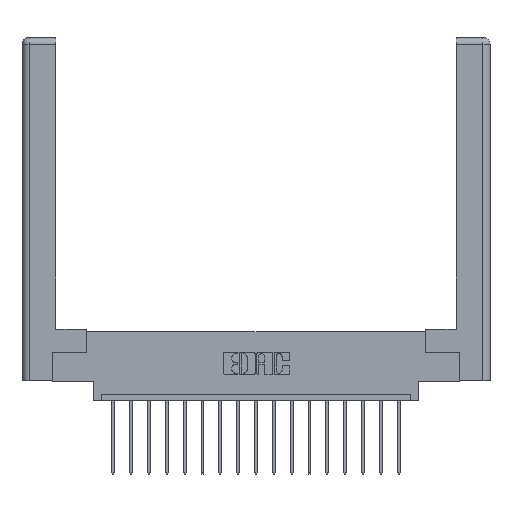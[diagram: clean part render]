
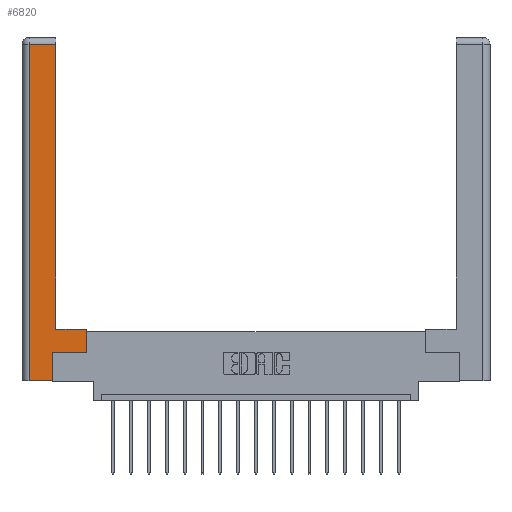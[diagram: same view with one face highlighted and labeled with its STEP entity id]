
A CAD part, top view. The second image highlights one B-rep face of the part: STEP entity #6820.
In plain terms, the highlighted planar face has unit normal (0, 0, 1).
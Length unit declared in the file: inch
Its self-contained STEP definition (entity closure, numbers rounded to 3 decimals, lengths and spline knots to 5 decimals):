
#52 = EDGE_CURVE ( 'NONE', #8139, #12732, #12989, .T. ) ;
#193 = DIRECTION ( 'NONE',  ( -1., 0., 0. ) ) ;
#220 = CARTESIAN_POINT ( 'NONE',  ( 0.565, 0.45, 0. ) ) ;
#452 = DIRECTION ( 'NONE',  ( 0., 1., 0. ) ) ;
#694 = EDGE_CURVE ( 'NONE', #10817, #9784, #9829, .T. ) ;
#1513 = VECTOR ( 'NONE', #9734, 39.37008 ) ;
#1611 = CARTESIAN_POINT ( 'NONE',  ( 0.295, 0.45, 0. ) ) ;
#1675 = ORIENTED_EDGE ( 'NONE', *, *, #2517, .T. ) ;
#1858 = VERTEX_POINT ( 'NONE', #13927 ) ;
#2036 = ORIENTED_EDGE ( 'NONE', *, *, #6158, .T. ) ;
#2280 = VECTOR ( 'NONE', #14547, 39.37008 ) ;
#2361 = EDGE_CURVE ( 'NONE', #12071, #10817, #10763, .T. ) ;
#2517 = EDGE_CURVE ( 'NONE', #3323, #8139, #18394, .T. ) ;
#2618 = VECTOR ( 'NONE', #4330, 39.37008 ) ;
#2687 = CARTESIAN_POINT ( 'NONE',  ( 0.265, 0., 0. ) ) ;
#3151 = EDGE_LOOP ( 'NONE', ( #13550, #15215, #8294, #9806, #11134, #3473, #2036, #1675 ) ) ;
#3323 = VERTEX_POINT ( 'NONE', #18029 ) ;
#3473 = ORIENTED_EDGE ( 'NONE', *, *, #9167, .T. ) ;
#3903 = DIRECTION ( 'NONE',  ( -1., 0., 0. ) ) ;
#3981 = DIRECTION ( 'NONE',  ( 0., -1., 0. ) ) ;
#4330 = DIRECTION ( 'NONE',  ( -1., 0., 0. ) ) ;
#4354 = CARTESIAN_POINT ( 'NONE',  ( 0.0615, 2.94, 0. ) ) ;
#4836 = LINE ( 'NONE', #7757, #17467 ) ;
#5787 = LINE ( 'NONE', #8100, #18199 ) ;
#5850 = CARTESIAN_POINT ( 'NONE',  ( 0., 0., 0. ) ) ;
#6158 = EDGE_CURVE ( 'NONE', #1858, #3323, #18065, .T. ) ;
#6314 = FACE_OUTER_BOUND ( 'NONE', #3151, .T. ) ;
#6737 = AXIS2_PLACEMENT_3D ( 'NONE', #5850, #15933, #193 ) ;
#6820 = ADVANCED_FACE ( 'NONE', ( #6314 ), #8842, .F. ) ;
#6875 = DIRECTION ( 'NONE',  ( 1., 0., 0. ) ) ;
#6959 = EDGE_CURVE ( 'NONE', #9784, #10483, #4836, .T. ) ;
#7757 = CARTESIAN_POINT ( 'NONE',  ( 0.265, 0.245, 0. ) ) ;
#7842 = VECTOR ( 'NONE', #6875, 39.37008 ) ;
#8068 = LINE ( 'NONE', #14029, #7842 ) ;
#8100 = CARTESIAN_POINT ( 'NONE',  ( 0.0615, 2.94, 0. ) ) ;
#8139 = VERTEX_POINT ( 'NONE', #1611 ) ;
#8294 = ORIENTED_EDGE ( 'NONE', *, *, #2361, .T. ) ;
#8742 = DIRECTION ( 'NONE',  ( 1., 0., 0. ) ) ;
#8842 = PLANE ( 'NONE',  #6737 ) ;
#9167 = EDGE_CURVE ( 'NONE', #10483, #1858, #8068, .T. ) ;
#9734 = DIRECTION ( 'NONE',  ( 0., 1., 0. ) ) ;
#9784 = VERTEX_POINT ( 'NONE', #2687 ) ;
#9806 = ORIENTED_EDGE ( 'NONE', *, *, #694, .T. ) ;
#9829 = LINE ( 'NONE', #17100, #16829 ) ;
#9892 = CARTESIAN_POINT ( 'NONE',  ( 0.0615, 0., 0. ) ) ;
#10483 = VERTEX_POINT ( 'NONE', #13160 ) ;
#10763 = LINE ( 'NONE', #15104, #12325 ) ;
#10817 = VERTEX_POINT ( 'NONE', #9892 ) ;
#11057 = CARTESIAN_POINT ( 'NONE',  ( 0.295, 3., 0. ) ) ;
#11134 = ORIENTED_EDGE ( 'NONE', *, *, #6959, .T. ) ;
#12071 = VERTEX_POINT ( 'NONE', #4354 ) ;
#12325 = VECTOR ( 'NONE', #3981, 39.37008 ) ;
#12732 = VERTEX_POINT ( 'NONE', #17029 ) ;
#12810 = CARTESIAN_POINT ( 'NONE',  ( 0.295, 0.45, 0. ) ) ;
#12989 = LINE ( 'NONE', #11057, #1513 ) ;
#13160 = CARTESIAN_POINT ( 'NONE',  ( 0.265, 0.245, 0. ) ) ;
#13550 = ORIENTED_EDGE ( 'NONE', *, *, #52, .T. ) ;
#13927 = CARTESIAN_POINT ( 'NONE',  ( 0.565, 0.245, 0. ) ) ;
#14029 = CARTESIAN_POINT ( 'NONE',  ( 0.565, 0.245, 0. ) ) ;
#14547 = DIRECTION ( 'NONE',  ( 0., 1., 0. ) ) ;
#15104 = CARTESIAN_POINT ( 'NONE',  ( 0.0615, 0., 0. ) ) ;
#15215 = ORIENTED_EDGE ( 'NONE', *, *, #16670, .T. ) ;
#15933 = DIRECTION ( 'NONE',  ( 0., 0., -1. ) ) ;
#16670 = EDGE_CURVE ( 'NONE', #12732, #12071, #5787, .T. ) ;
#16829 = VECTOR ( 'NONE', #8742, 39.37008 ) ;
#17029 = CARTESIAN_POINT ( 'NONE',  ( 0.295, 2.94, 0. ) ) ;
#17100 = CARTESIAN_POINT ( 'NONE',  ( 0.265, 0., 0. ) ) ;
#17467 = VECTOR ( 'NONE', #452, 39.37008 ) ;
#18029 = CARTESIAN_POINT ( 'NONE',  ( 0.565, 0.45, 0. ) ) ;
#18065 = LINE ( 'NONE', #220, #2280 ) ;
#18199 = VECTOR ( 'NONE', #3903, 39.37008 ) ;
#18394 = LINE ( 'NONE', #12810, #2618 ) ;
